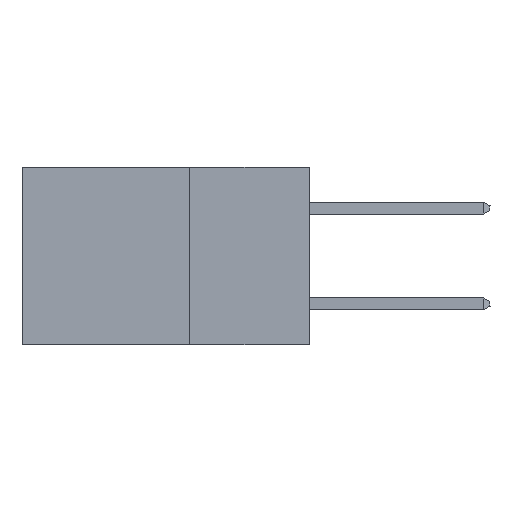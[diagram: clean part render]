
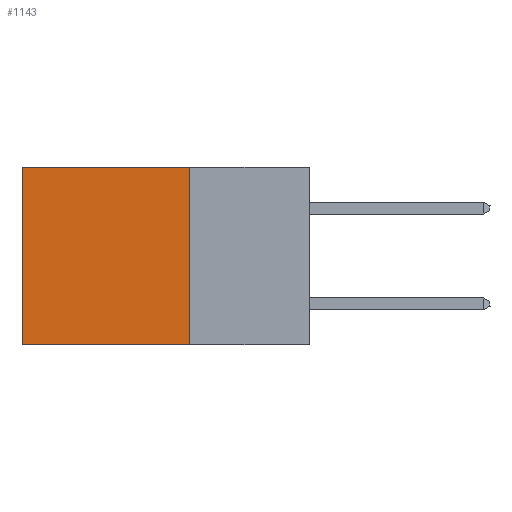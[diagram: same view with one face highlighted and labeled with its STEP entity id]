
A CAD part, left-side view. The second image highlights one B-rep face of the part: STEP entity #1143.
In plain terms, the highlighted planar face has unit normal (-1, 0, 0).
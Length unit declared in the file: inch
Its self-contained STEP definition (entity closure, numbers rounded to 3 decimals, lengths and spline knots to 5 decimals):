
#278 = VECTOR ( 'NONE', #18530, 39.37008 ) ;
#684 = ORIENTED_EDGE ( 'NONE', *, *, #12639, .F. ) ;
#689 = CARTESIAN_POINT ( 'NONE',  ( 0.2875, 0.6, 0. ) ) ;
#895 = VERTEX_POINT ( 'NONE', #1603 ) ;
#1143 = ADVANCED_FACE ( 'NONE', ( #1974 ), #18981, .F. ) ;
#1279 = LINE ( 'NONE', #689, #278 ) ;
#1603 = CARTESIAN_POINT ( 'NONE',  ( 0.2875, 0.25, 0. ) ) ;
#1680 = VERTEX_POINT ( 'NONE', #17649 ) ;
#1974 = FACE_OUTER_BOUND ( 'NONE', #15025, .T. ) ;
#4982 = DIRECTION ( 'NONE',  ( 0., 1., 0. ) ) ;
#5173 = VECTOR ( 'NONE', #4982, 39.37008 ) ;
#5760 = DIRECTION ( 'NONE',  ( 0., 0., -1. ) ) ;
#5946 = EDGE_CURVE ( 'NONE', #16578, #1680, #1279, .T. ) ;
#5973 = CARTESIAN_POINT ( 'NONE',  ( 0.2875, 0.25, 0. ) ) ;
#6450 = LINE ( 'NONE', #14754, #5173 ) ;
#8089 = DIRECTION ( 'NONE',  ( 0., 1., 0. ) ) ;
#8273 = VERTEX_POINT ( 'NONE', #14498 ) ;
#9065 = CARTESIAN_POINT ( 'NONE',  ( 0.2875, 0.6, 0. ) ) ;
#9078 = DIRECTION ( 'NONE',  ( 1., 0., 0. ) ) ;
#11199 = EDGE_CURVE ( 'NONE', #895, #16578, #18215, .T. ) ;
#11223 = CARTESIAN_POINT ( 'NONE',  ( 0.2875, 0.25, 0. ) ) ;
#12300 = EDGE_CURVE ( 'NONE', #895, #8273, #14112, .T. ) ;
#12506 = CARTESIAN_POINT ( 'NONE',  ( 0.2875, 0.25, 0. ) ) ;
#12639 = EDGE_CURVE ( 'NONE', #8273, #1680, #6450, .T. ) ;
#13888 = VECTOR ( 'NONE', #8089, 39.37008 ) ;
#13995 = DIRECTION ( 'NONE',  ( 0., 0., -1. ) ) ;
#14112 = LINE ( 'NONE', #5973, #16149 ) ;
#14498 = CARTESIAN_POINT ( 'NONE',  ( 0.2875, 0.25, -0.37 ) ) ;
#14754 = CARTESIAN_POINT ( 'NONE',  ( 0.2875, 0.25, -0.37 ) ) ;
#15025 = EDGE_LOOP ( 'NONE', ( #20861, #684, #20133, #16693 ) ) ;
#16149 = VECTOR ( 'NONE', #5760, 39.37008 ) ;
#16229 = AXIS2_PLACEMENT_3D ( 'NONE', #12506, #9078, #13995 ) ;
#16578 = VERTEX_POINT ( 'NONE', #9065 ) ;
#16693 = ORIENTED_EDGE ( 'NONE', *, *, #11199, .T. ) ;
#17649 = CARTESIAN_POINT ( 'NONE',  ( 0.2875, 0.6, -0.37 ) ) ;
#18215 = LINE ( 'NONE', #11223, #13888 ) ;
#18530 = DIRECTION ( 'NONE',  ( 0., 0., -1. ) ) ;
#18981 = PLANE ( 'NONE',  #16229 ) ;
#20133 = ORIENTED_EDGE ( 'NONE', *, *, #12300, .F. ) ;
#20861 = ORIENTED_EDGE ( 'NONE', *, *, #5946, .T. ) ;
